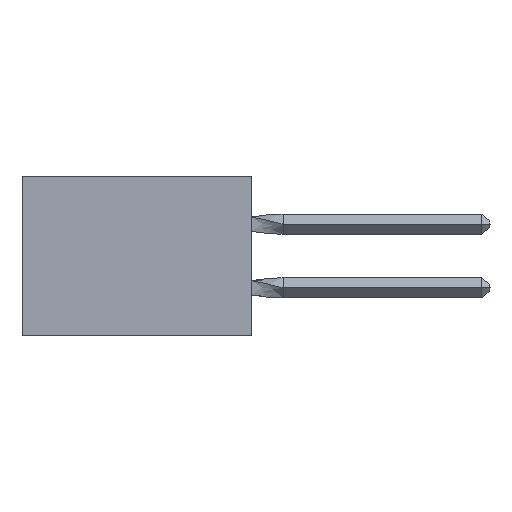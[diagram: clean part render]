
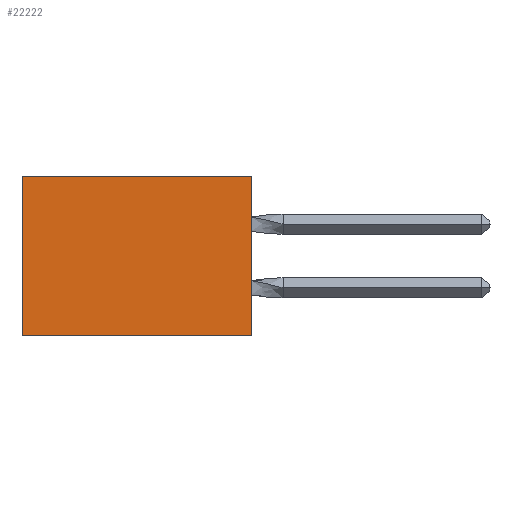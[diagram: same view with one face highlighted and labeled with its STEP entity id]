
A CAD part, left-side view. The second image highlights one B-rep face of the part: STEP entity #22222.
In plain terms, the highlighted planar face has unit normal (-1, 0, 0).
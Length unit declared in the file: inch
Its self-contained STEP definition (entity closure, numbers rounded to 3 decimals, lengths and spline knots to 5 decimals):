
#128 = LINE ( 'NONE', #9058, #29001 ) ;
#1034 = VECTOR ( 'NONE', #16816, 39.37008 ) ;
#1360 = DIRECTION ( 'NONE',  ( 0., 1., 0. ) ) ;
#1442 = CARTESIAN_POINT ( 'NONE',  ( 0.305, 0., 0. ) ) ;
#1644 = CARTESIAN_POINT ( 'NONE',  ( 0.305, 0.72, -0.5 ) ) ;
#3416 = ORIENTED_EDGE ( 'NONE', *, *, #18316, .T. ) ;
#3501 = DIRECTION ( 'NONE',  ( 0., 0., -1. ) ) ;
#3960 = AXIS2_PLACEMENT_3D ( 'NONE', #10671, #26779, #32944 ) ;
#4005 = VERTEX_POINT ( 'NONE', #15603 ) ;
#5206 = VERTEX_POINT ( 'NONE', #12881 ) ;
#6671 = ORIENTED_EDGE ( 'NONE', *, *, #7721, .F. ) ;
#6884 = VECTOR ( 'NONE', #9458, 39.37008 ) ;
#6952 = VERTEX_POINT ( 'NONE', #1644 ) ;
#7721 = EDGE_CURVE ( 'NONE', #5206, #23303, #18887, .T. ) ;
#9058 = CARTESIAN_POINT ( 'NONE',  ( 0.305, 0.72, -0.5 ) ) ;
#9323 = ORIENTED_EDGE ( 'NONE', *, *, #9579, .T. ) ;
#9458 = DIRECTION ( 'NONE',  ( 0., 0., -1. ) ) ;
#9579 = EDGE_CURVE ( 'NONE', #4005, #6952, #128, .T. ) ;
#10671 = CARTESIAN_POINT ( 'NONE',  ( 0.305, 0., -0.5 ) ) ;
#11467 = CARTESIAN_POINT ( 'NONE',  ( 0.305, 0., -0.5 ) ) ;
#12881 = CARTESIAN_POINT ( 'NONE',  ( 0.305, 0., 0. ) ) ;
#14005 = FACE_OUTER_BOUND ( 'NONE', #21859, .T. ) ;
#15326 = PLANE ( 'NONE',  #3960 ) ;
#15603 = CARTESIAN_POINT ( 'NONE',  ( 0.305, 0.72, 0. ) ) ;
#16816 = DIRECTION ( 'NONE',  ( 0., 1., 0. ) ) ;
#16834 = VECTOR ( 'NONE', #1360, 39.37008 ) ;
#17783 = ORIENTED_EDGE ( 'NONE', *, *, #31283, .F. ) ;
#18025 = LINE ( 'NONE', #1442, #1034 ) ;
#18316 = EDGE_CURVE ( 'NONE', #5206, #4005, #18025, .T. ) ;
#18887 = LINE ( 'NONE', #28096, #6884 ) ;
#21353 = LINE ( 'NONE', #27307, #16834 ) ;
#21859 = EDGE_LOOP ( 'NONE', ( #9323, #17783, #6671, #3416 ) ) ;
#22222 = ADVANCED_FACE ( 'NONE', ( #14005 ), #15326, .F. ) ;
#23303 = VERTEX_POINT ( 'NONE', #11467 ) ;
#26779 = DIRECTION ( 'NONE',  ( 1., 0., 0. ) ) ;
#27307 = CARTESIAN_POINT ( 'NONE',  ( 0.305, 0., -0.5 ) ) ;
#28096 = CARTESIAN_POINT ( 'NONE',  ( 0.305, 0., -0.5 ) ) ;
#29001 = VECTOR ( 'NONE', #3501, 39.37008 ) ;
#31283 = EDGE_CURVE ( 'NONE', #23303, #6952, #21353, .T. ) ;
#32944 = DIRECTION ( 'NONE',  ( 0., 0., -1. ) ) ;
